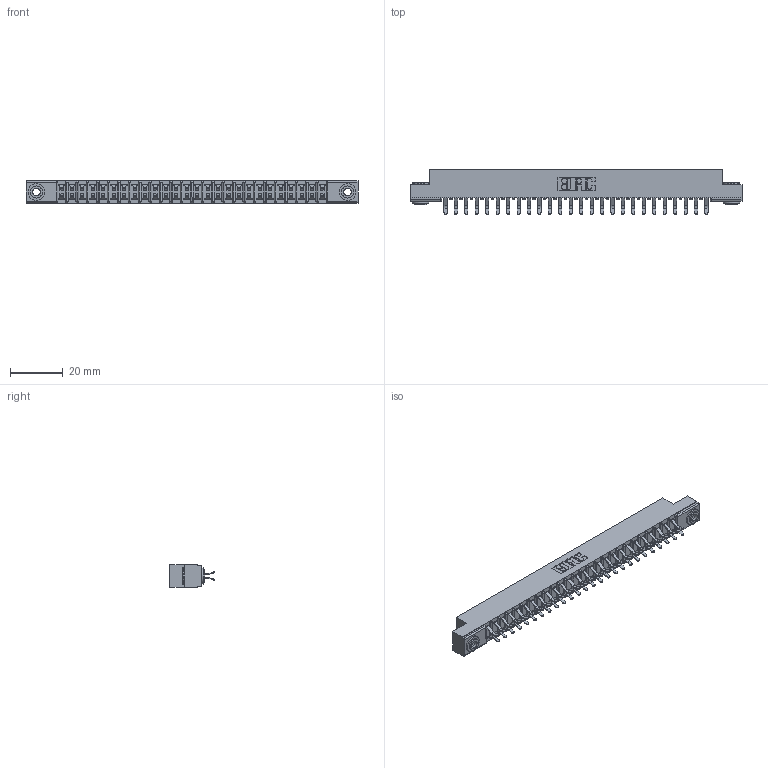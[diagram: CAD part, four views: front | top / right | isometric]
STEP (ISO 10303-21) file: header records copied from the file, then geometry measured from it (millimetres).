
FILE_DESCRIPTION (( 'STEP AP203' ), '1' );
FILE_NAME ('357-052-556-203.STEP', '2019-09-19T03:31:35', ( '' ), ( '' ), 'SwSTEP 2.0', 'SolidWorks 2016', '' );
FILE_SCHEMA (( 'CONFIG_CONTROL_DESIGN' ));
Length unit declared in the file: inch
Products named in the file (4): 345-250-002_345-250-002-102; 307 Part_.156 Dia Mounting Holes; 357-052-556-203; 307-290-001_556
Assembly tree (55 placements, depth 2):
  357-052-556-203
    307 Part_.156 Dia Mounting Holes
    307-290-001_556  x52
    345-250-002_345-250-002-102  x2
Bounding box: 126.03 x 16.97 x 8.71 mm (x, y, z)
Volume: 8235.4 mm3; surface area: 14949.7 mm2
Topology: 55 solids, 55 shells, 2797 faces, 7819 edges, 5066 vertices
Faces by surface type: plane 1810, cylinder 925, sphere 54, cone 8
Entity records: 26263 total; most frequent: CARTESIAN_POINT 4283, ORIENTED_EDGE 4234, DIRECTION 4217, EDGE_CURVE 2117, LINE 1609, VECTOR 1609, VERTEX_POINT 1370, AXIS2_PLACEMENT_3D 1304
